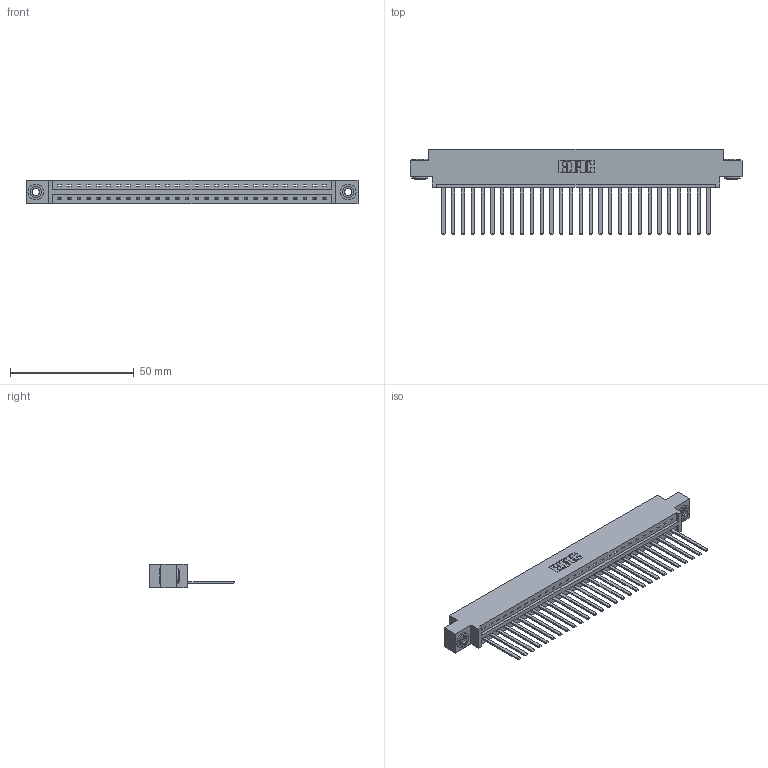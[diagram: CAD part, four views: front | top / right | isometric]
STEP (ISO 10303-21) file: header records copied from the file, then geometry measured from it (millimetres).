
FILE_DESCRIPTION (( 'STEP AP203' ), '1' );
FILE_NAME ('387-028-544-603.STEP', '2019-10-03T16:32:45', ( '' ), ( '' ), 'SwSTEP 2.0', 'SolidWorks 2016', '' );
FILE_SCHEMA (( 'CONFIG_CONTROL_DESIGN' ));
Length unit declared in the file: inch
Products named in the file (4): 387-028-544-603; 337 Part_0.170 Offset - 0.156 Dia-TH; 345-250-002_345-250-002-102; 345-292-001_345-293-144
Assembly tree (31 placements, depth 2):
  387-028-544-603
    337 Part_0.170 Offset - 0.156 Dia-TH
    345-292-001_345-293-144  x28
    345-250-002_345-250-002-102  x2
Bounding box: 133.96 x 34.3 x 9.4 mm (x, y, z)
Volume: 13973.8 mm3; surface area: 15758 mm2
Topology: 31 solids, 31 shells, 1724 faces, 5159 edges, 3398 vertices
Faces by surface type: plane 1260, cylinder 456, cone 8
Entity records: 23222 total; most frequent: CARTESIAN_POINT 4021, ORIENTED_EDGE 3978, DIRECTION 3443, EDGE_CURVE 1989, VECTOR 1841, LINE 1841, VERTEX_POINT 1322, AXIS2_PLACEMENT_3D 801
